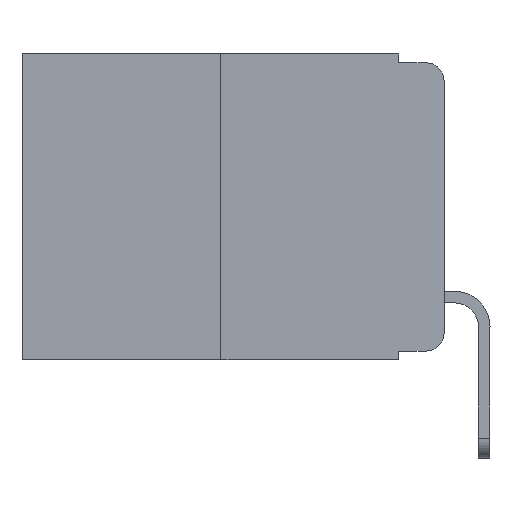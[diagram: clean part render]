
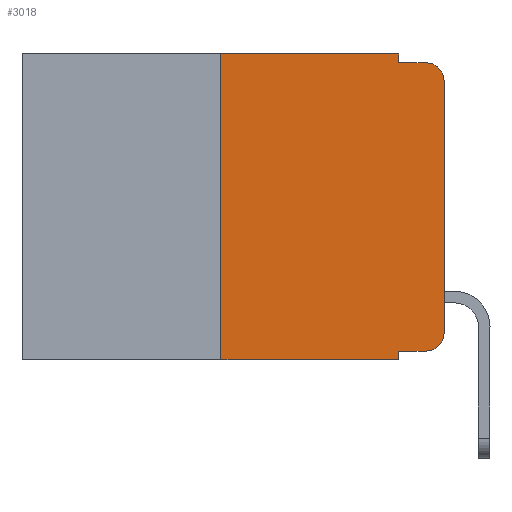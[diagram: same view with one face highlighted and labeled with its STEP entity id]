
A CAD part, left-side view. The second image highlights one B-rep face of the part: STEP entity #3018.
In plain terms, the highlighted planar face has unit normal (-1, 0, 0).
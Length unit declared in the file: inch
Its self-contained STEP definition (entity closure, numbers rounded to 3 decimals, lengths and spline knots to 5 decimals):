
#56 = VERTEX_POINT ( 'NONE', #8442 ) ;
#106 = VERTEX_POINT ( 'NONE', #734 ) ;
#226 = CARTESIAN_POINT ( 'NONE',  ( 0., 0.02, -0.03 ) ) ;
#540 = CARTESIAN_POINT ( 'NONE',  ( 0., 0.051, 0. ) ) ;
#734 = CARTESIAN_POINT ( 'NONE',  ( 0., 0.051, -0.343 ) ) ;
#867 = LINE ( 'NONE', #1665, #8725 ) ;
#905 = ORIENTED_EDGE ( 'NONE', *, *, #10108, .T. ) ;
#909 = DIRECTION ( 'NONE',  ( 0., 0., -1. ) ) ;
#1027 = VECTOR ( 'NONE', #4135, 39.37008 ) ;
#1046 = FACE_OUTER_BOUND ( 'NONE', #7057, .T. ) ;
#1334 = DIRECTION ( 'NONE',  ( 0., 0., -1. ) ) ;
#1562 = LINE ( 'NONE', #8909, #12378 ) ;
#1665 = CARTESIAN_POINT ( 'NONE',  ( 0., 0.25, 0. ) ) ;
#1850 = VERTEX_POINT ( 'NONE', #6462 ) ;
#1924 = LINE ( 'NONE', #7823, #4411 ) ;
#2048 = LINE ( 'NONE', #8533, #4191 ) ;
#2112 = CARTESIAN_POINT ( 'NONE',  ( 0., 0.051, -0.333 ) ) ;
#2285 = CARTESIAN_POINT ( 'NONE',  ( 0., 0., -0.313 ) ) ;
#2397 = AXIS2_PLACEMENT_3D ( 'NONE', #9176, #9103, #9072 ) ;
#2845 = CARTESIAN_POINT ( 'NONE',  ( 0., 0.02, -0.01 ) ) ;
#3018 = ADVANCED_FACE ( 'NONE', ( #1046 ), #9235, .F. ) ;
#3265 = LINE ( 'NONE', #2112, #5438 ) ;
#3441 = LINE ( 'NONE', #540, #11097 ) ;
#3600 = LINE ( 'NONE', #12460, #1027 ) ;
#3614 = CIRCLE ( 'NONE', #6582, 0.02 ) ;
#3784 = DIRECTION ( 'NONE',  ( 0., 0., -1. ) ) ;
#4114 = ORIENTED_EDGE ( 'NONE', *, *, #10212, .F. ) ;
#4135 = DIRECTION ( 'NONE',  ( 0., -1., 0. ) ) ;
#4191 = VECTOR ( 'NONE', #9575, 39.37008 ) ;
#4346 = DIRECTION ( 'NONE',  ( 0., 0., 1. ) ) ;
#4411 = VECTOR ( 'NONE', #6823, 39.37008 ) ;
#4626 = ORIENTED_EDGE ( 'NONE', *, *, #10603, .F. ) ;
#5211 = VERTEX_POINT ( 'NONE', #8140 ) ;
#5438 = VECTOR ( 'NONE', #10511, 39.37008 ) ;
#5545 = CARTESIAN_POINT ( 'NONE',  ( 0., 0.02, -0.333 ) ) ;
#6462 = CARTESIAN_POINT ( 'NONE',  ( 0., 0.051, 0. ) ) ;
#6465 = LINE ( 'NONE', #6528, #9853 ) ;
#6502 = AXIS2_PLACEMENT_3D ( 'NONE', #13449, #7350, #909 ) ;
#6528 = CARTESIAN_POINT ( 'NONE',  ( 0., 0., 0. ) ) ;
#6582 = AXIS2_PLACEMENT_3D ( 'NONE', #226, #7744, #1334 ) ;
#6717 = ORIENTED_EDGE ( 'NONE', *, *, #11338, .T. ) ;
#6823 = DIRECTION ( 'NONE',  ( 0., -1., 0. ) ) ;
#6846 = CARTESIAN_POINT ( 'NONE',  ( 0., 0., -0.03 ) ) ;
#7057 = EDGE_LOOP ( 'NONE', ( #11788, #905, #4114, #7142, #4626, #10192, #11142, #9071, #7535, #6717 ) ) ;
#7142 = ORIENTED_EDGE ( 'NONE', *, *, #10231, .F. ) ;
#7339 = VERTEX_POINT ( 'NONE', #6846 ) ;
#7350 = DIRECTION ( 'NONE',  ( -1., 0., 0. ) ) ;
#7382 = CARTESIAN_POINT ( 'NONE',  ( 0., 0.25, 0. ) ) ;
#7535 = ORIENTED_EDGE ( 'NONE', *, *, #10671, .T. ) ;
#7744 = DIRECTION ( 'NONE',  ( -1., 0., 0. ) ) ;
#7823 = CARTESIAN_POINT ( 'NONE',  ( 0., 0.051, -0.01 ) ) ;
#7862 = DIRECTION ( 'NONE',  ( 0., 0., -1. ) ) ;
#8140 = CARTESIAN_POINT ( 'NONE',  ( 0., 0.051, -0.01 ) ) ;
#8310 = VERTEX_POINT ( 'NONE', #7382 ) ;
#8442 = CARTESIAN_POINT ( 'NONE',  ( 0., 0.25, -0.343 ) ) ;
#8533 = CARTESIAN_POINT ( 'NONE',  ( 0., 0.473, -0.343 ) ) ;
#8725 = VECTOR ( 'NONE', #9069, 39.37008 ) ;
#8909 = CARTESIAN_POINT ( 'NONE',  ( 0., 0.051, 0. ) ) ;
#9069 = DIRECTION ( 'NONE',  ( 0., 0., 1. ) ) ;
#9071 = ORIENTED_EDGE ( 'NONE', *, *, #10343, .F. ) ;
#9072 = DIRECTION ( 'NONE',  ( 0., 0., -1. ) ) ;
#9103 = DIRECTION ( 'NONE',  ( 1., 0., 0. ) ) ;
#9176 = CARTESIAN_POINT ( 'NONE',  ( 0., 0.473, 0. ) ) ;
#9235 = PLANE ( 'NONE',  #2397 ) ;
#9374 = VERTEX_POINT ( 'NONE', #12299 ) ;
#9575 = DIRECTION ( 'NONE',  ( 0., -1., 0. ) ) ;
#9608 = EDGE_CURVE ( 'NONE', #13280, #7339, #6465, .T. ) ;
#9853 = VECTOR ( 'NONE', #4346, 39.37008 ) ;
#10108 = EDGE_CURVE ( 'NONE', #7339, #12796, #3614, .T. ) ;
#10192 = ORIENTED_EDGE ( 'NONE', *, *, #10325, .F. ) ;
#10212 = EDGE_CURVE ( 'NONE', #5211, #12796, #1924, .T. ) ;
#10231 = EDGE_CURVE ( 'NONE', #1850, #5211, #1562, .T. ) ;
#10325 = EDGE_CURVE ( 'NONE', #56, #8310, #867, .T. ) ;
#10343 = EDGE_CURVE ( 'NONE', #9374, #106, #3441, .T. ) ;
#10511 = DIRECTION ( 'NONE',  ( 0., -1., 0. ) ) ;
#10603 = EDGE_CURVE ( 'NONE', #8310, #1850, #3600, .T. ) ;
#10671 = EDGE_CURVE ( 'NONE', #9374, #11963, #3265, .T. ) ;
#11097 = VECTOR ( 'NONE', #3784, 39.37008 ) ;
#11142 = ORIENTED_EDGE ( 'NONE', *, *, #12462, .T. ) ;
#11338 = EDGE_CURVE ( 'NONE', #11963, #13280, #12346, .T. ) ;
#11788 = ORIENTED_EDGE ( 'NONE', *, *, #9608, .T. ) ;
#11963 = VERTEX_POINT ( 'NONE', #5545 ) ;
#12299 = CARTESIAN_POINT ( 'NONE',  ( 0., 0.051, -0.333 ) ) ;
#12346 = CIRCLE ( 'NONE', #6502, 0.02 ) ;
#12378 = VECTOR ( 'NONE', #7862, 39.37008 ) ;
#12460 = CARTESIAN_POINT ( 'NONE',  ( 0., 0.473, 0. ) ) ;
#12462 = EDGE_CURVE ( 'NONE', #56, #106, #2048, .T. ) ;
#12796 = VERTEX_POINT ( 'NONE', #2845 ) ;
#13280 = VERTEX_POINT ( 'NONE', #2285 ) ;
#13449 = CARTESIAN_POINT ( 'NONE',  ( 0., 0.02, -0.313 ) ) ;
